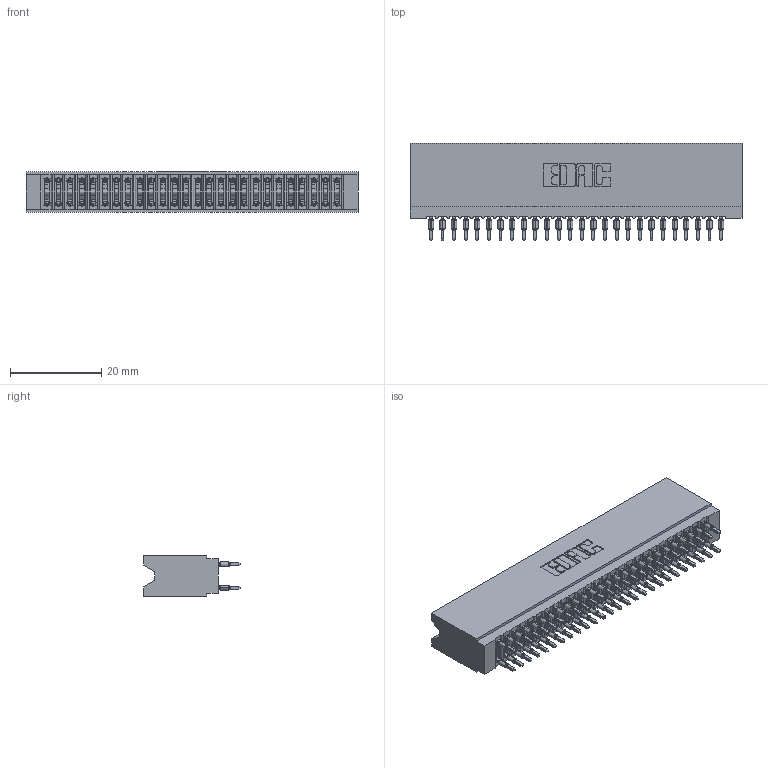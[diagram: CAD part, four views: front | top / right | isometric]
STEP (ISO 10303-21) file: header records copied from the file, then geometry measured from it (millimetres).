
FILE_DESCRIPTION (( 'STEP AP203' ), '1' );
FILE_NAME ('745-052-560-206.STEP', '2020-09-12T05:57:41', ( '' ), ( '' ), 'SwSTEP 2.0', 'SolidWorks 2020', '' );
FILE_SCHEMA (( 'CONFIG_CONTROL_DESIGN' ));
Length unit declared in the file: inch
Products named in the file (3): 745-052-560-206; 745-292-001_560; 745 Part_Insulator Option - 06
Assembly tree (53 placements, depth 2):
  745-052-560-206
    745 Part_Insulator Option - 06
    745-292-001_560  x52
Bounding box: 72.64 x 21.22 x 8.89 mm (x, y, z)
Volume: 6808.7 mm3; surface area: 14318.6 mm2
Topology: 53 solids, 53 shells, 5218 faces, 14274 edges, 9064 vertices
Faces by surface type: plane 2708, cylinder 1158, bspline 1040, torus 312
Entity records: 46305 total; most frequent: CARTESIAN_POINT 8540, ORIENTED_EDGE 7944, DIRECTION 6958, EDGE_CURVE 3972, LINE 3626, VECTOR 3626, VERTEX_POINT 2536, AXIS2_PLACEMENT_3D 1666
